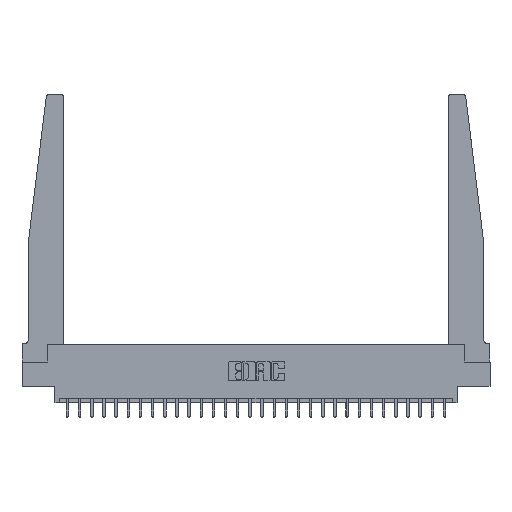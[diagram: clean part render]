
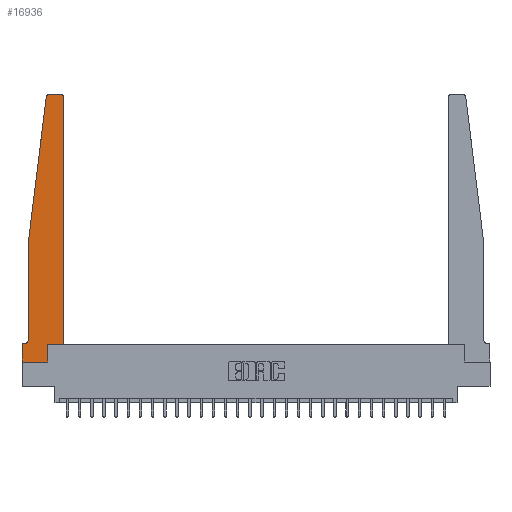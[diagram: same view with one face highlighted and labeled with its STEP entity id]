
A CAD part, top view. The second image highlights one B-rep face of the part: STEP entity #16936.
In plain terms, the highlighted planar face has unit normal (0, 0, 1).
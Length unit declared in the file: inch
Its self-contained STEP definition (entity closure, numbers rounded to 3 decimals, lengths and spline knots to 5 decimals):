
#99 = EDGE_CURVE ( 'NONE', #885, #4357, #22061, .T. ) ;
#605 = CIRCLE ( 'NONE', #16659, 0.03 ) ;
#853 = VECTOR ( 'NONE', #23031, 39.37008 ) ;
#885 = VERTEX_POINT ( 'NONE', #8720 ) ;
#1101 = VERTEX_POINT ( 'NONE', #27174 ) ;
#1160 = ORIENTED_EDGE ( 'NONE', *, *, #11909, .T. ) ;
#1626 = CIRCLE ( 'NONE', #13617, 0.05 ) ;
#1880 = VECTOR ( 'NONE', #22052, 39.37008 ) ;
#2283 = VECTOR ( 'NONE', #20394, 39.37008 ) ;
#3335 = VERTEX_POINT ( 'NONE', #16744 ) ;
#3456 = CARTESIAN_POINT ( 'NONE',  ( 0.065, 1.25, 0.37 ) ) ;
#3464 = LINE ( 'NONE', #22150, #26814 ) ;
#3515 = EDGE_CURVE ( 'NONE', #10963, #885, #18518, .T. ) ;
#3755 = FACE_OUTER_BOUND ( 'NONE', #26414, .T. ) ;
#4357 = VERTEX_POINT ( 'NONE', #10620 ) ;
#4705 = EDGE_CURVE ( 'NONE', #25461, #19158, #12986, .T. ) ;
#4742 = ORIENTED_EDGE ( 'NONE', *, *, #22814, .T. ) ;
#4968 = CARTESIAN_POINT ( 'NONE',  ( 0., 0., 0.37 ) ) ;
#5048 = CARTESIAN_POINT ( 'NONE',  ( 0.015, 0.2375, 0.37 ) ) ;
#5085 = ORIENTED_EDGE ( 'NONE', *, *, #99, .T. ) ;
#5140 = VERTEX_POINT ( 'NONE', #25248 ) ;
#5553 = CARTESIAN_POINT ( 'NONE',  ( 0.425, 0.18, 0.37 ) ) ;
#5605 = CARTESIAN_POINT ( 'NONE',  ( 0.27653, 2.72, 0.37 ) ) ;
#5918 = ORIENTED_EDGE ( 'NONE', *, *, #9571, .T. ) ;
#6142 = ORIENTED_EDGE ( 'NONE', *, *, #4705, .T. ) ;
#6146 = VERTEX_POINT ( 'NONE', #9194 ) ;
#6763 = DIRECTION ( 'NONE',  ( 0., 0., 1. ) ) ;
#6978 = EDGE_CURVE ( 'NONE', #4357, #20172, #605, .T. ) ;
#7361 = EDGE_CURVE ( 'NONE', #20172, #25461, #10110, .T. ) ;
#7499 = LINE ( 'NONE', #22163, #22577 ) ;
#7925 = AXIS2_PLACEMENT_3D ( 'NONE', #18672, #12775, #19354 ) ;
#8519 = AXIS2_PLACEMENT_3D ( 'NONE', #5605, #18164, #12001 ) ;
#8720 = CARTESIAN_POINT ( 'NONE',  ( 0.425, 0.18, 0.37 ) ) ;
#8922 = DIRECTION ( 'NONE',  ( 0., 0., -1. ) ) ;
#9194 = CARTESIAN_POINT ( 'NONE',  ( 0.2605, 0., 0.37 ) ) ;
#9571 = EDGE_CURVE ( 'NONE', #5140, #1101, #1626, .T. ) ;
#9911 = LINE ( 'NONE', #13819, #2283 ) ;
#9923 = LINE ( 'NONE', #18439, #853 ) ;
#10110 = LINE ( 'NONE', #24920, #21140 ) ;
#10155 = PLANE ( 'NONE',  #7925 ) ;
#10620 = CARTESIAN_POINT ( 'NONE',  ( 0.425, 2.72, 0.37 ) ) ;
#10768 = ORIENTED_EDGE ( 'NONE', *, *, #6978, .T. ) ;
#10963 = VERTEX_POINT ( 'NONE', #26828 ) ;
#11257 = DIRECTION ( 'NONE',  ( -0.122, -0.992, 0. ) ) ;
#11683 = VECTOR ( 'NONE', #14190, 39.37008 ) ;
#11909 = EDGE_CURVE ( 'NONE', #19158, #13126, #7499, .T. ) ;
#11926 = DIRECTION ( 'NONE',  ( 0., -1., 0. ) ) ;
#12001 = DIRECTION ( 'NONE',  ( 1., 0., 0. ) ) ;
#12775 = DIRECTION ( 'NONE',  ( 0., 0., 1. ) ) ;
#12957 = ORIENTED_EDGE ( 'NONE', *, *, #3515, .T. ) ;
#12986 = CIRCLE ( 'NONE', #8519, 0.03 ) ;
#13126 = VERTEX_POINT ( 'NONE', #21174 ) ;
#13617 = AXIS2_PLACEMENT_3D ( 'NONE', #5048, #8922, #19832 ) ;
#13819 = CARTESIAN_POINT ( 'NONE',  ( 0., 0., 0.37 ) ) ;
#14190 = DIRECTION ( 'NONE',  ( 1., 0., 0. ) ) ;
#15193 = LINE ( 'NONE', #23731, #1880 ) ;
#15850 = ORIENTED_EDGE ( 'NONE', *, *, #17234, .T. ) ;
#16114 = EDGE_CURVE ( 'NONE', #3335, #20441, #9911, .T. ) ;
#16659 = AXIS2_PLACEMENT_3D ( 'NONE', #19468, #6763, #19608 ) ;
#16744 = CARTESIAN_POINT ( 'NONE',  ( 0., 0.1875, 0.37 ) ) ;
#16936 = ADVANCED_FACE ( 'NONE', ( #3755 ), #10155, .T. ) ;
#17234 = EDGE_CURVE ( 'NONE', #13126, #5140, #23091, .T. ) ;
#18164 = DIRECTION ( 'NONE',  ( 0., 0., 1. ) ) ;
#18439 = CARTESIAN_POINT ( 'NONE',  ( 0.2605, 0.18, 0.37 ) ) ;
#18484 = DIRECTION ( 'NONE',  ( -1., 0., 0. ) ) ;
#18518 = LINE ( 'NONE', #5553, #11683 ) ;
#18672 = CARTESIAN_POINT ( 'NONE',  ( 0., 0.1875, 0.37 ) ) ;
#19158 = VERTEX_POINT ( 'NONE', #24325 ) ;
#19340 = VECTOR ( 'NONE', #26129, 39.37008 ) ;
#19354 = DIRECTION ( 'NONE',  ( 1., 0., 0. ) ) ;
#19396 = EDGE_CURVE ( 'NONE', #6146, #10963, #9923, .T. ) ;
#19468 = CARTESIAN_POINT ( 'NONE',  ( 0.395, 2.72, 0.37 ) ) ;
#19608 = DIRECTION ( 'NONE',  ( 1., 0., 0. ) ) ;
#19677 = ORIENTED_EDGE ( 'NONE', *, *, #7361, .T. ) ;
#19832 = DIRECTION ( 'NONE',  ( -1., 0., 0. ) ) ;
#20172 = VERTEX_POINT ( 'NONE', #24532 ) ;
#20213 = CARTESIAN_POINT ( 'NONE',  ( 0.27653, 2.75, 0.37 ) ) ;
#20394 = DIRECTION ( 'NONE',  ( 0., -1., 0. ) ) ;
#20441 = VERTEX_POINT ( 'NONE', #4968 ) ;
#20899 = VECTOR ( 'NONE', #11926, 39.37008 ) ;
#21140 = VECTOR ( 'NONE', #18484, 39.37008 ) ;
#21174 = CARTESIAN_POINT ( 'NONE',  ( 0.065, 1.25, 0.37 ) ) ;
#21768 = CARTESIAN_POINT ( 'NONE',  ( 0.425, 0.18, 0.37 ) ) ;
#22034 = EDGE_CURVE ( 'NONE', #20441, #6146, #3464, .T. ) ;
#22052 = DIRECTION ( 'NONE',  ( -1., 0., 0. ) ) ;
#22061 = LINE ( 'NONE', #21768, #19340 ) ;
#22150 = CARTESIAN_POINT ( 'NONE',  ( 0., 0., 0.37 ) ) ;
#22163 = CARTESIAN_POINT ( 'NONE',  ( 0.065, 1.25, 0.37 ) ) ;
#22577 = VECTOR ( 'NONE', #11257, 39.37008 ) ;
#22814 = EDGE_CURVE ( 'NONE', #1101, #3335, #15193, .T. ) ;
#23031 = DIRECTION ( 'NONE',  ( 0., 1., 0. ) ) ;
#23091 = LINE ( 'NONE', #3456, #20899 ) ;
#23584 = ORIENTED_EDGE ( 'NONE', *, *, #22034, .T. ) ;
#23731 = CARTESIAN_POINT ( 'NONE',  ( 0.065, 0.1875, 0.37 ) ) ;
#24325 = CARTESIAN_POINT ( 'NONE',  ( 0.24675, 2.72367, 0.37 ) ) ;
#24532 = CARTESIAN_POINT ( 'NONE',  ( 0.395, 2.75, 0.37 ) ) ;
#24706 = ORIENTED_EDGE ( 'NONE', *, *, #19396, .T. ) ;
#24920 = CARTESIAN_POINT ( 'NONE',  ( 0.25, 2.75, 0.37 ) ) ;
#25248 = CARTESIAN_POINT ( 'NONE',  ( 0.065, 0.2375, 0.37 ) ) ;
#25461 = VERTEX_POINT ( 'NONE', #20213 ) ;
#26129 = DIRECTION ( 'NONE',  ( 0., 1., 0. ) ) ;
#26414 = EDGE_LOOP ( 'NONE', ( #19677, #6142, #1160, #15850, #5918, #4742, #26678, #23584, #24706, #12957, #5085, #10768 ) ) ;
#26678 = ORIENTED_EDGE ( 'NONE', *, *, #16114, .T. ) ;
#26779 = DIRECTION ( 'NONE',  ( 1., 0., 0. ) ) ;
#26814 = VECTOR ( 'NONE', #26779, 39.37008 ) ;
#26828 = CARTESIAN_POINT ( 'NONE',  ( 0.2605, 0.18, 0.37 ) ) ;
#27174 = CARTESIAN_POINT ( 'NONE',  ( 0.015, 0.1875, 0.37 ) ) ;
